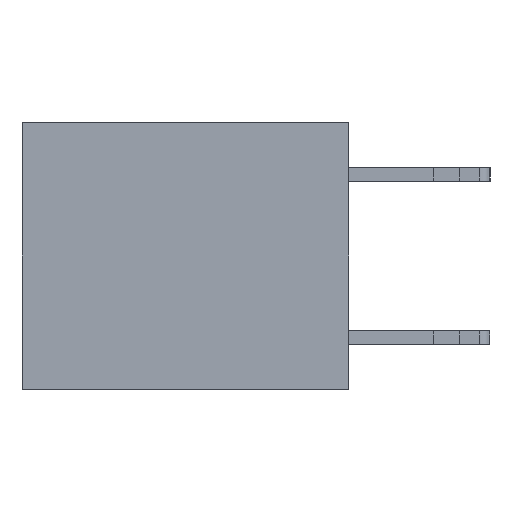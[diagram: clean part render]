
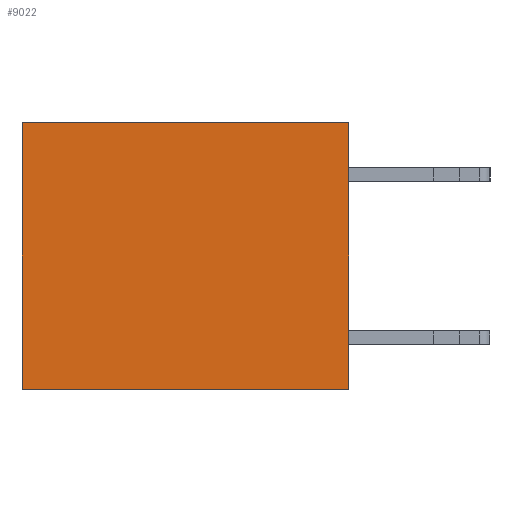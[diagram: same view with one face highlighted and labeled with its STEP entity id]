
A CAD part, left-side view. The second image highlights one B-rep face of the part: STEP entity #9022.
In plain terms, the highlighted planar face has unit normal (-1, 0, 0).
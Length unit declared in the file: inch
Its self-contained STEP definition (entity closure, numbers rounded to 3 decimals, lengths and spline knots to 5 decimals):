
#508 = CARTESIAN_POINT ( 'NONE',  ( 0.3165, 0., 0. ) ) ;
#1925 = LINE ( 'NONE', #14548, #10742 ) ;
#2254 = EDGE_CURVE ( 'NONE', #12755, #8760, #1925, .T. ) ;
#2490 = LINE ( 'NONE', #14946, #16397 ) ;
#2740 = CARTESIAN_POINT ( 'NONE',  ( 0.3165, 0.6, -0.49 ) ) ;
#3564 = EDGE_CURVE ( 'NONE', #12041, #5919, #2490, .T. ) ;
#4102 = ORIENTED_EDGE ( 'NONE', *, *, #3564, .F. ) ;
#4403 = LINE ( 'NONE', #12281, #11585 ) ;
#4672 = CARTESIAN_POINT ( 'NONE',  ( 0.3165, 0.6, 0. ) ) ;
#5339 = CARTESIAN_POINT ( 'NONE',  ( 0.3165, 0., -0.49 ) ) ;
#5919 = VERTEX_POINT ( 'NONE', #5339 ) ;
#6729 = FACE_OUTER_BOUND ( 'NONE', #7067, .T. ) ;
#7067 = EDGE_LOOP ( 'NONE', ( #13512, #13899, #4102, #9596 ) ) ;
#7828 = PLANE ( 'NONE',  #13314 ) ;
#8760 = VERTEX_POINT ( 'NONE', #2740 ) ;
#8793 = DIRECTION ( 'NONE',  ( 0., 1., 0. ) ) ;
#9022 = ADVANCED_FACE ( 'NONE', ( #6729 ), #7828, .F. ) ;
#9188 = CARTESIAN_POINT ( 'NONE',  ( 0.3165, 0., -0.49 ) ) ;
#9596 = ORIENTED_EDGE ( 'NONE', *, *, #16091, .T. ) ;
#10574 = DIRECTION ( 'NONE',  ( 1., 0., 0. ) ) ;
#10742 = VECTOR ( 'NONE', #11834, 39.37008 ) ;
#11366 = CARTESIAN_POINT ( 'NONE',  ( 0.3165, 0., -0.49 ) ) ;
#11585 = VECTOR ( 'NONE', #13771, 39.37008 ) ;
#11834 = DIRECTION ( 'NONE',  ( 0., 0., -1. ) ) ;
#12041 = VERTEX_POINT ( 'NONE', #508 ) ;
#12281 = CARTESIAN_POINT ( 'NONE',  ( 0.3165, 0., 0. ) ) ;
#12755 = VERTEX_POINT ( 'NONE', #4672 ) ;
#13314 = AXIS2_PLACEMENT_3D ( 'NONE', #9188, #10574, #17086 ) ;
#13512 = ORIENTED_EDGE ( 'NONE', *, *, #2254, .T. ) ;
#13560 = DIRECTION ( 'NONE',  ( 0., 0., -1. ) ) ;
#13771 = DIRECTION ( 'NONE',  ( 0., 1., 0. ) ) ;
#13899 = ORIENTED_EDGE ( 'NONE', *, *, #15121, .F. ) ;
#14548 = CARTESIAN_POINT ( 'NONE',  ( 0.3165, 0.6, -0.49 ) ) ;
#14781 = LINE ( 'NONE', #11366, #17336 ) ;
#14946 = CARTESIAN_POINT ( 'NONE',  ( 0.3165, 0., -0.49 ) ) ;
#15121 = EDGE_CURVE ( 'NONE', #5919, #8760, #14781, .T. ) ;
#16091 = EDGE_CURVE ( 'NONE', #12041, #12755, #4403, .T. ) ;
#16397 = VECTOR ( 'NONE', #13560, 39.37008 ) ;
#17086 = DIRECTION ( 'NONE',  ( 0., 0., -1. ) ) ;
#17336 = VECTOR ( 'NONE', #8793, 39.37008 ) ;
